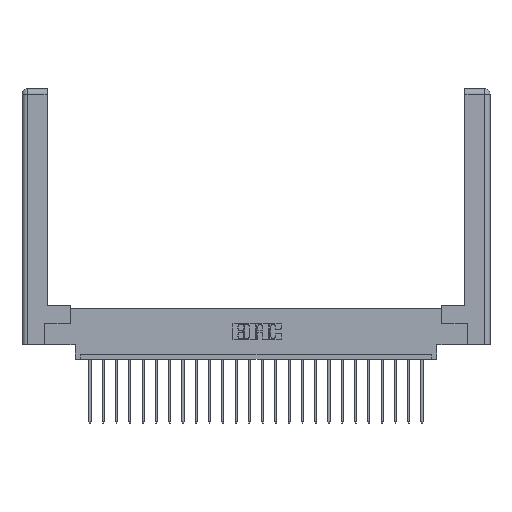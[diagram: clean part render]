
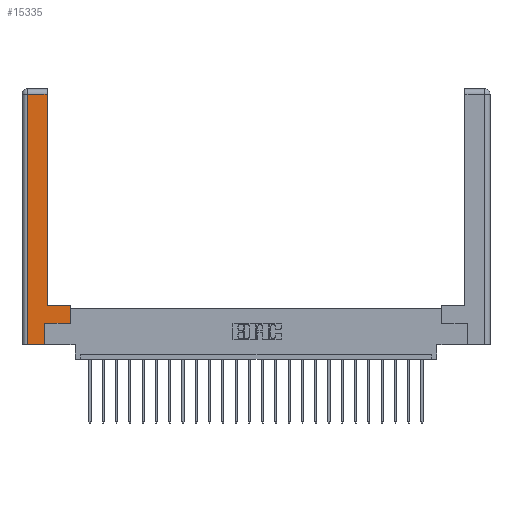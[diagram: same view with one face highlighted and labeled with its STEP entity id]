
A CAD part, top view. The second image highlights one B-rep face of the part: STEP entity #15335.
In plain terms, the highlighted planar face has unit normal (0, 0, 1).
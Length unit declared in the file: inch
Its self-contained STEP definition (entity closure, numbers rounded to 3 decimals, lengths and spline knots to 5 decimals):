
#908 = LINE ( 'NONE', #20416, #17253 ) ;
#1972 = VECTOR ( 'NONE', #5430, 39.37008 ) ;
#2137 = ORIENTED_EDGE ( 'NONE', *, *, #18016, .T. ) ;
#2665 = CARTESIAN_POINT ( 'NONE',  ( 0.565, 0.245, 0. ) ) ;
#2795 = LINE ( 'NONE', #16353, #22079 ) ;
#3390 = DIRECTION ( 'NONE',  ( -1., 0., 0. ) ) ;
#3664 = EDGE_CURVE ( 'NONE', #13006, #14560, #16874, .T. ) ;
#4075 = DIRECTION ( 'NONE',  ( 0., 1., 0. ) ) ;
#5430 = DIRECTION ( 'NONE',  ( 0., 1., 0. ) ) ;
#5631 = VERTEX_POINT ( 'NONE', #21789 ) ;
#5677 = EDGE_CURVE ( 'NONE', #5631, #19060, #9196, .T. ) ;
#6741 = CARTESIAN_POINT ( 'NONE',  ( 0.565, 0.45, 0. ) ) ;
#7489 = CARTESIAN_POINT ( 'NONE',  ( 0.265, 0., 0. ) ) ;
#8525 = DIRECTION ( 'NONE',  ( -1., 0., 0. ) ) ;
#8948 = EDGE_LOOP ( 'NONE', ( #18963, #14513, #2137, #23989, #20435, #16653, #13810, #10872 ) ) ;
#9196 = LINE ( 'NONE', #10868, #16169 ) ;
#9712 = VECTOR ( 'NONE', #4075, 39.37008 ) ;
#10234 = PLANE ( 'NONE',  #18984 ) ;
#10638 = DIRECTION ( 'NONE',  ( -1., 0., 0. ) ) ;
#10868 = CARTESIAN_POINT ( 'NONE',  ( 0.0615, 2.94, 0. ) ) ;
#10872 = ORIENTED_EDGE ( 'NONE', *, *, #22963, .T. ) ;
#11394 = EDGE_CURVE ( 'NONE', #16227, #13825, #2795, .T. ) ;
#11483 = LINE ( 'NONE', #19143, #17284 ) ;
#12219 = EDGE_CURVE ( 'NONE', #13825, #22823, #23117, .T. ) ;
#12954 = CARTESIAN_POINT ( 'NONE',  ( 0.565, 0.45, 0. ) ) ;
#13006 = VERTEX_POINT ( 'NONE', #2665 ) ;
#13810 = ORIENTED_EDGE ( 'NONE', *, *, #3664, .T. ) ;
#13825 = VERTEX_POINT ( 'NONE', #7489 ) ;
#13908 = LINE ( 'NONE', #22086, #20267 ) ;
#14513 = ORIENTED_EDGE ( 'NONE', *, *, #5677, .T. ) ;
#14560 = VERTEX_POINT ( 'NONE', #6741 ) ;
#14864 = CARTESIAN_POINT ( 'NONE',  ( 0.295, 0.45, 0. ) ) ;
#15335 = ADVANCED_FACE ( 'NONE', ( #17696 ), #10234, .F. ) ;
#15787 = CARTESIAN_POINT ( 'NONE',  ( 0., 0., 0. ) ) ;
#16169 = VECTOR ( 'NONE', #10638, 39.37008 ) ;
#16227 = VERTEX_POINT ( 'NONE', #20949 ) ;
#16353 = CARTESIAN_POINT ( 'NONE',  ( 0.265, 0., 0. ) ) ;
#16653 = ORIENTED_EDGE ( 'NONE', *, *, #16669, .T. ) ;
#16669 = EDGE_CURVE ( 'NONE', #22823, #13006, #13908, .T. ) ;
#16874 = LINE ( 'NONE', #12954, #1972 ) ;
#17253 = VECTOR ( 'NONE', #3390, 39.37008 ) ;
#17284 = VECTOR ( 'NONE', #19393, 39.37008 ) ;
#17340 = VERTEX_POINT ( 'NONE', #14864 ) ;
#17696 = FACE_OUTER_BOUND ( 'NONE', #8948, .T. ) ;
#18016 = EDGE_CURVE ( 'NONE', #19060, #16227, #11483, .T. ) ;
#18736 = CARTESIAN_POINT ( 'NONE',  ( 0.265, 0.245, 0. ) ) ;
#18963 = ORIENTED_EDGE ( 'NONE', *, *, #21337, .T. ) ;
#18984 = AXIS2_PLACEMENT_3D ( 'NONE', #15787, #19652, #8525 ) ;
#19060 = VERTEX_POINT ( 'NONE', #22394 ) ;
#19143 = CARTESIAN_POINT ( 'NONE',  ( 0.0615, 0., 0. ) ) ;
#19393 = DIRECTION ( 'NONE',  ( 0., -1., 0. ) ) ;
#19652 = DIRECTION ( 'NONE',  ( 0., 0., -1. ) ) ;
#19729 = CARTESIAN_POINT ( 'NONE',  ( 0.295, 3., 0. ) ) ;
#20101 = DIRECTION ( 'NONE',  ( 1., 0., 0. ) ) ;
#20267 = VECTOR ( 'NONE', #20101, 39.37008 ) ;
#20416 = CARTESIAN_POINT ( 'NONE',  ( 0.295, 0.45, 0. ) ) ;
#20435 = ORIENTED_EDGE ( 'NONE', *, *, #12219, .T. ) ;
#20949 = CARTESIAN_POINT ( 'NONE',  ( 0.0615, 0., 0. ) ) ;
#21337 = EDGE_CURVE ( 'NONE', #17340, #5631, #22300, .T. ) ;
#21713 = DIRECTION ( 'NONE',  ( 0., 1., 0. ) ) ;
#21789 = CARTESIAN_POINT ( 'NONE',  ( 0.295, 2.94, 0. ) ) ;
#22068 = CARTESIAN_POINT ( 'NONE',  ( 0.265, 0.245, 0. ) ) ;
#22079 = VECTOR ( 'NONE', #23853, 39.37008 ) ;
#22086 = CARTESIAN_POINT ( 'NONE',  ( 0.565, 0.245, 0. ) ) ;
#22300 = LINE ( 'NONE', #19729, #22567 ) ;
#22394 = CARTESIAN_POINT ( 'NONE',  ( 0.0615, 2.94, 0. ) ) ;
#22567 = VECTOR ( 'NONE', #21713, 39.37008 ) ;
#22823 = VERTEX_POINT ( 'NONE', #22068 ) ;
#22963 = EDGE_CURVE ( 'NONE', #14560, #17340, #908, .T. ) ;
#23117 = LINE ( 'NONE', #18736, #9712 ) ;
#23853 = DIRECTION ( 'NONE',  ( 1., 0., 0. ) ) ;
#23989 = ORIENTED_EDGE ( 'NONE', *, *, #11394, .T. ) ;
